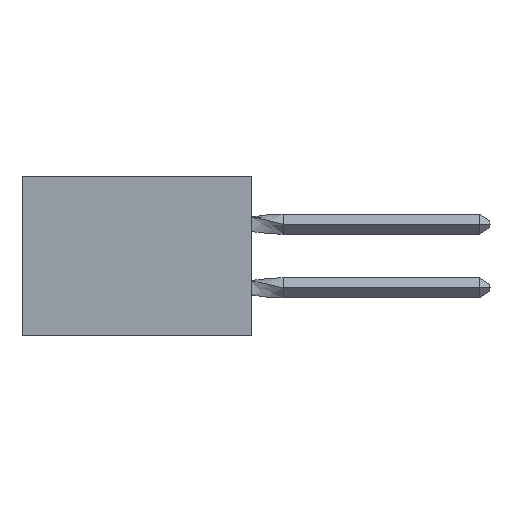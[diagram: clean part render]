
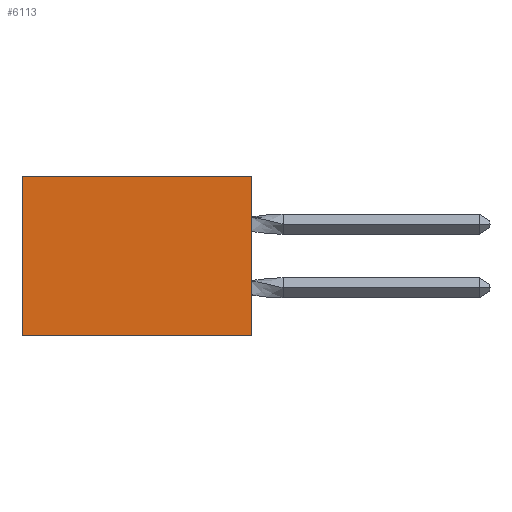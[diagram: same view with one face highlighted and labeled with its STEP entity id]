
A CAD part, left-side view. The second image highlights one B-rep face of the part: STEP entity #6113.
In plain terms, the highlighted planar face has unit normal (-1, 0, 0).
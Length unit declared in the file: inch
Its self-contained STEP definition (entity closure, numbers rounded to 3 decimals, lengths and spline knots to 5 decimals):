
#127 = CARTESIAN_POINT ( 'NONE',  ( 0.305, 0.72, -0.5 ) ) ;
#506 = CARTESIAN_POINT ( 'NONE',  ( 0.305, 0.72, 0. ) ) ;
#543 = PLANE ( 'NONE',  #15428 ) ;
#766 = VECTOR ( 'NONE', #16456, 39.37008 ) ;
#1612 = CARTESIAN_POINT ( 'NONE',  ( 0.305, 0., -0.5 ) ) ;
#1797 = CARTESIAN_POINT ( 'NONE',  ( 0.305, 0., -0.5 ) ) ;
#1837 = CARTESIAN_POINT ( 'NONE',  ( 0.305, 0., -0.5 ) ) ;
#3446 = ORIENTED_EDGE ( 'NONE', *, *, #5427, .T. ) ;
#3511 = CARTESIAN_POINT ( 'NONE',  ( 0.305, 0., 0. ) ) ;
#3917 = EDGE_LOOP ( 'NONE', ( #3446, #14354, #6473, #11991 ) ) ;
#4565 = LINE ( 'NONE', #1612, #766 ) ;
#5427 = EDGE_CURVE ( 'NONE', #9936, #13064, #11916, .T. ) ;
#6113 = ADVANCED_FACE ( 'NONE', ( #12315 ), #543, .F. ) ;
#6473 = ORIENTED_EDGE ( 'NONE', *, *, #11600, .F. ) ;
#6867 = CARTESIAN_POINT ( 'NONE',  ( 0.305, 0., -0.5 ) ) ;
#7264 = DIRECTION ( 'NONE',  ( 0., 1., 0. ) ) ;
#8392 = VERTEX_POINT ( 'NONE', #6867 ) ;
#8423 = LINE ( 'NONE', #3511, #15157 ) ;
#8706 = DIRECTION ( 'NONE',  ( 1., 0., 0. ) ) ;
#9936 = VERTEX_POINT ( 'NONE', #506 ) ;
#11296 = DIRECTION ( 'NONE',  ( 0., 0., -1. ) ) ;
#11600 = EDGE_CURVE ( 'NONE', #13502, #8392, #4565, .T. ) ;
#11916 = LINE ( 'NONE', #15494, #13605 ) ;
#11991 = ORIENTED_EDGE ( 'NONE', *, *, #17081, .T. ) ;
#12315 = FACE_OUTER_BOUND ( 'NONE', #3917, .T. ) ;
#13064 = VERTEX_POINT ( 'NONE', #127 ) ;
#13118 = DIRECTION ( 'NONE',  ( 0., 0., -1. ) ) ;
#13468 = EDGE_CURVE ( 'NONE', #8392, #13064, #14424, .T. ) ;
#13502 = VERTEX_POINT ( 'NONE', #16873 ) ;
#13605 = VECTOR ( 'NONE', #13118, 39.37008 ) ;
#14354 = ORIENTED_EDGE ( 'NONE', *, *, #13468, .F. ) ;
#14424 = LINE ( 'NONE', #1797, #16980 ) ;
#15157 = VECTOR ( 'NONE', #16931, 39.37008 ) ;
#15428 = AXIS2_PLACEMENT_3D ( 'NONE', #1837, #8706, #11296 ) ;
#15494 = CARTESIAN_POINT ( 'NONE',  ( 0.305, 0.72, -0.5 ) ) ;
#16456 = DIRECTION ( 'NONE',  ( 0., 0., -1. ) ) ;
#16873 = CARTESIAN_POINT ( 'NONE',  ( 0.305, 0., 0. ) ) ;
#16931 = DIRECTION ( 'NONE',  ( 0., 1., 0. ) ) ;
#16980 = VECTOR ( 'NONE', #7264, 39.37008 ) ;
#17081 = EDGE_CURVE ( 'NONE', #13502, #9936, #8423, .T. ) ;
